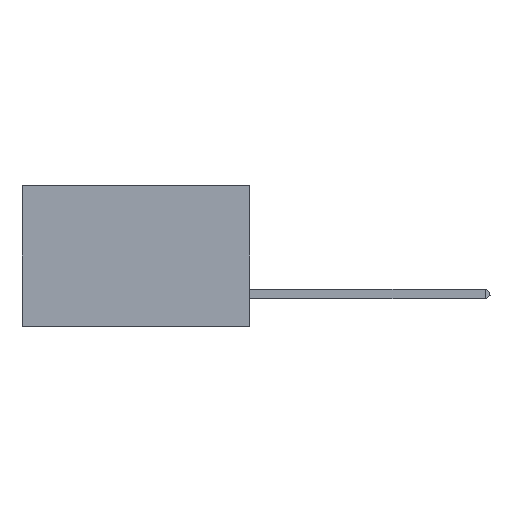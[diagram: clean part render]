
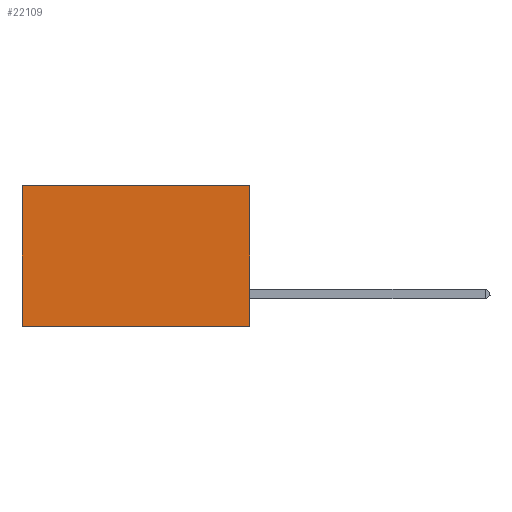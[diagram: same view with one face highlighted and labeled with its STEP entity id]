
A CAD part, left-side view. The second image highlights one B-rep face of the part: STEP entity #22109.
In plain terms, the highlighted planar face has unit normal (-1, 0, 0).
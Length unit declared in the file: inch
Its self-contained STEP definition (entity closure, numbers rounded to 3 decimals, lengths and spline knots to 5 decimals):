
#842 = VERTEX_POINT ( 'NONE', #8199 ) ;
#1303 = CARTESIAN_POINT ( 'NONE',  ( 0.2875, 0., 0. ) ) ;
#2312 = LINE ( 'NONE', #19163, #3572 ) ;
#3572 = VECTOR ( 'NONE', #13097, 39.37008 ) ;
#4852 = LINE ( 'NONE', #9798, #18586 ) ;
#5630 = PLANE ( 'NONE',  #14583 ) ;
#5710 = DIRECTION ( 'NONE',  ( 0., 0., -1. ) ) ;
#6011 = EDGE_LOOP ( 'NONE', ( #8439, #13410, #18031, #16126 ) ) ;
#6996 = EDGE_CURVE ( 'NONE', #25879, #842, #23133, .T. ) ;
#7735 = EDGE_CURVE ( 'NONE', #11764, #842, #4852, .T. ) ;
#8199 = CARTESIAN_POINT ( 'NONE',  ( 0.2875, 0.6, -0.37 ) ) ;
#8439 = ORIENTED_EDGE ( 'NONE', *, *, #7735, .T. ) ;
#8999 = CARTESIAN_POINT ( 'NONE',  ( 0.2875, 0., -0.37 ) ) ;
#9798 = CARTESIAN_POINT ( 'NONE',  ( 0.2875, 0.6, 0. ) ) ;
#11196 = DIRECTION ( 'NONE',  ( 0., 1., 0. ) ) ;
#11667 = CARTESIAN_POINT ( 'NONE',  ( 0.2875, 0., -0.37 ) ) ;
#11764 = VERTEX_POINT ( 'NONE', #25151 ) ;
#12312 = VECTOR ( 'NONE', #11196, 39.37008 ) ;
#13097 = DIRECTION ( 'NONE',  ( 0., 1., 0. ) ) ;
#13107 = EDGE_CURVE ( 'NONE', #16776, #11764, #2312, .T. ) ;
#13410 = ORIENTED_EDGE ( 'NONE', *, *, #6996, .F. ) ;
#13540 = EDGE_CURVE ( 'NONE', #16776, #25879, #18584, .T. ) ;
#14583 = AXIS2_PLACEMENT_3D ( 'NONE', #15906, #22191, #5710 ) ;
#15906 = CARTESIAN_POINT ( 'NONE',  ( 0.2875, 0., 0. ) ) ;
#16126 = ORIENTED_EDGE ( 'NONE', *, *, #13107, .T. ) ;
#16647 = CARTESIAN_POINT ( 'NONE',  ( 0.2875, 0., 0. ) ) ;
#16776 = VERTEX_POINT ( 'NONE', #1303 ) ;
#17299 = FACE_OUTER_BOUND ( 'NONE', #6011, .T. ) ;
#17830 = DIRECTION ( 'NONE',  ( 0., 0., -1. ) ) ;
#18031 = ORIENTED_EDGE ( 'NONE', *, *, #13540, .F. ) ;
#18584 = LINE ( 'NONE', #16647, #24314 ) ;
#18586 = VECTOR ( 'NONE', #17830, 39.37008 ) ;
#19163 = CARTESIAN_POINT ( 'NONE',  ( 0.2875, 0., 0. ) ) ;
#22109 = ADVANCED_FACE ( 'NONE', ( #17299 ), #5630, .F. ) ;
#22191 = DIRECTION ( 'NONE',  ( 1., 0., 0. ) ) ;
#22971 = DIRECTION ( 'NONE',  ( 0., 0., -1. ) ) ;
#23133 = LINE ( 'NONE', #8999, #12312 ) ;
#24314 = VECTOR ( 'NONE', #22971, 39.37008 ) ;
#25151 = CARTESIAN_POINT ( 'NONE',  ( 0.2875, 0.6, 0. ) ) ;
#25879 = VERTEX_POINT ( 'NONE', #11667 ) ;
